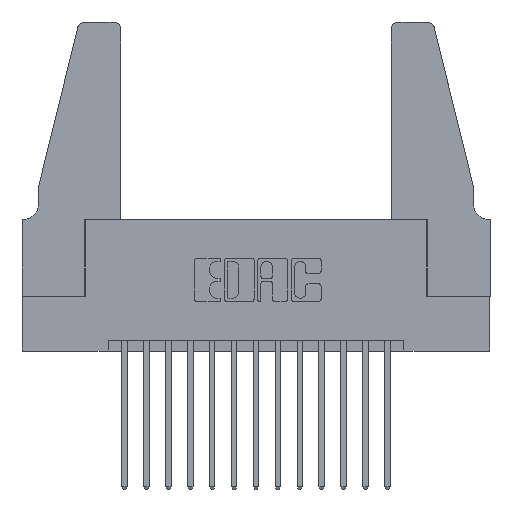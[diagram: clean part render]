
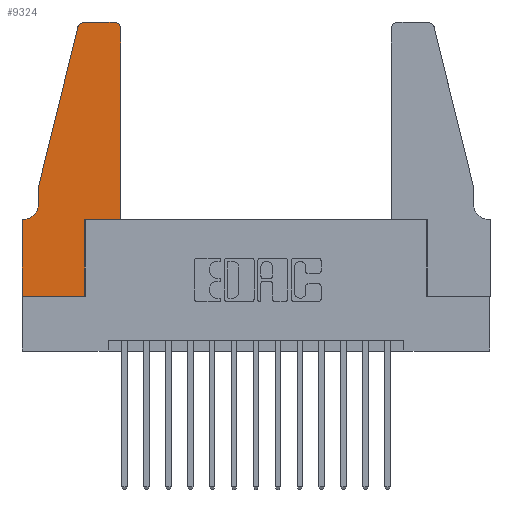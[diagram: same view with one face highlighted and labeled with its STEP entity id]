
A CAD part, top view. The second image highlights one B-rep face of the part: STEP entity #9324.
In plain terms, the highlighted planar face has unit normal (0, 0, 1).
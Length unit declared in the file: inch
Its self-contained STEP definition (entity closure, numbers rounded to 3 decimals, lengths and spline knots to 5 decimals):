
#46 = ORIENTED_EDGE ( 'NONE', *, *, #5295, .T. ) ;
#86 = LINE ( 'NONE', #9310, #5621 ) ;
#203 = AXIS2_PLACEMENT_3D ( 'NONE', #15200, #12730, #14296 ) ;
#204 = CARTESIAN_POINT ( 'NONE',  ( 0.25487, 1.22718, 0.37 ) ) ;
#671 = DIRECTION ( 'NONE',  ( 1., 0., 0. ) ) ;
#694 = DIRECTION ( 'NONE',  ( 1., 0., 0. ) ) ;
#926 = VECTOR ( 'NONE', #13490, 39.37008 ) ;
#972 = DIRECTION ( 'NONE',  ( 0., 0., 1. ) ) ;
#1044 = VERTEX_POINT ( 'NONE', #1560 ) ;
#1107 = DIRECTION ( 'NONE',  ( 0., -1., 0. ) ) ;
#1189 = EDGE_CURVE ( 'NONE', #12129, #4324, #4047, .T. ) ;
#1379 = ORIENTED_EDGE ( 'NONE', *, *, #8104, .T. ) ;
#1503 = CARTESIAN_POINT ( 'NONE',  ( 0.4505, 1.22, 0.37 ) ) ;
#1560 = CARTESIAN_POINT ( 'NONE',  ( 0.0755, 0.42, 0.37 ) ) ;
#1601 = EDGE_CURVE ( 'NONE', #4324, #8514, #11746, .T. ) ;
#1618 = ORIENTED_EDGE ( 'NONE', *, *, #10933, .T. ) ;
#2095 = CARTESIAN_POINT ( 'NONE',  ( 0.0755, 0.5, 0.37 ) ) ;
#2262 = PLANE ( 'NONE',  #5814 ) ;
#2329 = CARTESIAN_POINT ( 'NONE',  ( 0., 0., 0.37 ) ) ;
#2961 = DIRECTION ( 'NONE',  ( -1., 0., 0. ) ) ;
#2991 = EDGE_CURVE ( 'NONE', #7412, #9613, #86, .T. ) ;
#3022 = DIRECTION ( 'NONE',  ( 0., 0., -1. ) ) ;
#3097 = DIRECTION ( 'NONE',  ( 1., 0., 0. ) ) ;
#3192 = AXIS2_PLACEMENT_3D ( 'NONE', #9193, #3022, #2961 ) ;
#3255 = DIRECTION ( 'NONE',  ( 0., 1., 0. ) ) ;
#3396 = CIRCLE ( 'NONE', #203, 0.03 ) ;
#3453 = ORIENTED_EDGE ( 'NONE', *, *, #14962, .T. ) ;
#3805 = VERTEX_POINT ( 'NONE', #14614 ) ;
#4047 = LINE ( 'NONE', #15688, #11733 ) ;
#4240 = CARTESIAN_POINT ( 'NONE',  ( 0.0055, 0.35, 0.37 ) ) ;
#4324 = VERTEX_POINT ( 'NONE', #13986 ) ;
#4479 = AXIS2_PLACEMENT_3D ( 'NONE', #13044, #10599, #3097 ) ;
#4485 = VECTOR ( 'NONE', #15983, 39.37008 ) ;
#4496 = CARTESIAN_POINT ( 'NONE',  ( 0., 0., 0.37 ) ) ;
#4637 = EDGE_CURVE ( 'NONE', #3805, #11873, #8066, .T. ) ;
#4683 = DIRECTION ( 'NONE',  ( 1., 0., 0. ) ) ;
#5295 = EDGE_CURVE ( 'NONE', #1044, #9697, #6506, .T. ) ;
#5316 = ORIENTED_EDGE ( 'NONE', *, *, #6608, .T. ) ;
#5455 = DIRECTION ( 'NONE',  ( -1., 0., 0. ) ) ;
#5621 = VECTOR ( 'NONE', #5455, 39.37008 ) ;
#5814 = AXIS2_PLACEMENT_3D ( 'NONE', #5846, #972, #4683 ) ;
#5846 = CARTESIAN_POINT ( 'NONE',  ( 0., 0.35, 0.37 ) ) ;
#5864 = LINE ( 'NONE', #15147, #926 ) ;
#6506 = CIRCLE ( 'NONE', #3192, 0.07 ) ;
#6608 = EDGE_CURVE ( 'NONE', #9488, #1044, #5864, .T. ) ;
#7244 = DIRECTION ( 'NONE',  ( -1., 0., 0. ) ) ;
#7412 = VERTEX_POINT ( 'NONE', #14067 ) ;
#7522 = EDGE_CURVE ( 'NONE', #9697, #3805, #16053, .T. ) ;
#7566 = VECTOR ( 'NONE', #9469, 39.37008 ) ;
#7580 = VECTOR ( 'NONE', #7244, 39.37008 ) ;
#7588 = ORIENTED_EDGE ( 'NONE', *, *, #1189, .T. ) ;
#7800 = LINE ( 'NONE', #2095, #4485 ) ;
#8066 = LINE ( 'NONE', #8636, #13417 ) ;
#8104 = EDGE_CURVE ( 'NONE', #10868, #12129, #12059, .T. ) ;
#8440 = EDGE_CURVE ( 'NONE', #8514, #7412, #3396, .T. ) ;
#8514 = VERTEX_POINT ( 'NONE', #1503 ) ;
#8636 = CARTESIAN_POINT ( 'NONE',  ( 0., 0., 0.37 ) ) ;
#8692 = ORIENTED_EDGE ( 'NONE', *, *, #1601, .T. ) ;
#8906 = VECTOR ( 'NONE', #694, 39.37008 ) ;
#9020 = FACE_OUTER_BOUND ( 'NONE', #15612, .T. ) ;
#9193 = CARTESIAN_POINT ( 'NONE',  ( 0.0055, 0.42, 0.37 ) ) ;
#9265 = ORIENTED_EDGE ( 'NONE', *, *, #2991, .T. ) ;
#9310 = CARTESIAN_POINT ( 'NONE',  ( 0.2605, 1.25, 0.37 ) ) ;
#9324 = ADVANCED_FACE ( 'NONE', ( #9020 ), #2262, .T. ) ;
#9469 = DIRECTION ( 'NONE',  ( 0., 1., 0. ) ) ;
#9488 = VERTEX_POINT ( 'NONE', #12478 ) ;
#9496 = LINE ( 'NONE', #4496, #8906 ) ;
#9613 = VERTEX_POINT ( 'NONE', #12801 ) ;
#9697 = VERTEX_POINT ( 'NONE', #4240 ) ;
#10599 = DIRECTION ( 'NONE',  ( 0., 0., 1. ) ) ;
#10868 = VERTEX_POINT ( 'NONE', #13253 ) ;
#10907 = CARTESIAN_POINT ( 'NONE',  ( 0.4505, 0.35, 0.37 ) ) ;
#10933 = EDGE_CURVE ( 'NONE', #12591, #9488, #7800, .T. ) ;
#10987 = CARTESIAN_POINT ( 'NONE',  ( 0.0755, 0.35, 0.37 ) ) ;
#11659 = CIRCLE ( 'NONE', #4479, 0.03 ) ;
#11733 = VECTOR ( 'NONE', #671, 39.37008 ) ;
#11746 = LINE ( 'NONE', #10907, #7566 ) ;
#11873 = VERTEX_POINT ( 'NONE', #2329 ) ;
#12059 = LINE ( 'NONE', #12088, #14794 ) ;
#12088 = CARTESIAN_POINT ( 'NONE',  ( 0.2865, 0.35, 0.37 ) ) ;
#12129 = VERTEX_POINT ( 'NONE', #15400 ) ;
#12232 = ORIENTED_EDGE ( 'NONE', *, *, #8440, .T. ) ;
#12478 = CARTESIAN_POINT ( 'NONE',  ( 0.0755, 0.5, 0.37 ) ) ;
#12591 = VERTEX_POINT ( 'NONE', #204 ) ;
#12730 = DIRECTION ( 'NONE',  ( 0., 0., 1. ) ) ;
#12801 = CARTESIAN_POINT ( 'NONE',  ( 0.284, 1.25, 0.37 ) ) ;
#12968 = EDGE_CURVE ( 'NONE', #11873, #10868, #9496, .T. ) ;
#13044 = CARTESIAN_POINT ( 'NONE',  ( 0.284, 1.22, 0.37 ) ) ;
#13178 = ORIENTED_EDGE ( 'NONE', *, *, #7522, .T. ) ;
#13253 = CARTESIAN_POINT ( 'NONE',  ( 0.2865, 0., 0.37 ) ) ;
#13417 = VECTOR ( 'NONE', #1107, 39.37008 ) ;
#13420 = ORIENTED_EDGE ( 'NONE', *, *, #12968, .T. ) ;
#13490 = DIRECTION ( 'NONE',  ( 0., -1., 0. ) ) ;
#13986 = CARTESIAN_POINT ( 'NONE',  ( 0.4505, 0.35, 0.37 ) ) ;
#14067 = CARTESIAN_POINT ( 'NONE',  ( 0.4205, 1.25, 0.37 ) ) ;
#14296 = DIRECTION ( 'NONE',  ( 1., 0., 0. ) ) ;
#14614 = CARTESIAN_POINT ( 'NONE',  ( 0., 0.35, 0.37 ) ) ;
#14794 = VECTOR ( 'NONE', #3255, 39.37008 ) ;
#14962 = EDGE_CURVE ( 'NONE', #9613, #12591, #11659, .T. ) ;
#15147 = CARTESIAN_POINT ( 'NONE',  ( 0.0755, 0.5, 0.37 ) ) ;
#15200 = CARTESIAN_POINT ( 'NONE',  ( 0.4205, 1.22, 0.37 ) ) ;
#15320 = ORIENTED_EDGE ( 'NONE', *, *, #4637, .T. ) ;
#15400 = CARTESIAN_POINT ( 'NONE',  ( 0.2865, 0.35, 0.37 ) ) ;
#15612 = EDGE_LOOP ( 'NONE', ( #9265, #3453, #1618, #5316, #46, #13178, #15320, #13420, #1379, #7588, #8692, #12232 ) ) ;
#15688 = CARTESIAN_POINT ( 'NONE',  ( 0.4505, 0.35, 0.37 ) ) ;
#15983 = DIRECTION ( 'NONE',  ( -0.239, -0.971, 0. ) ) ;
#16053 = LINE ( 'NONE', #10987, #7580 ) ;
